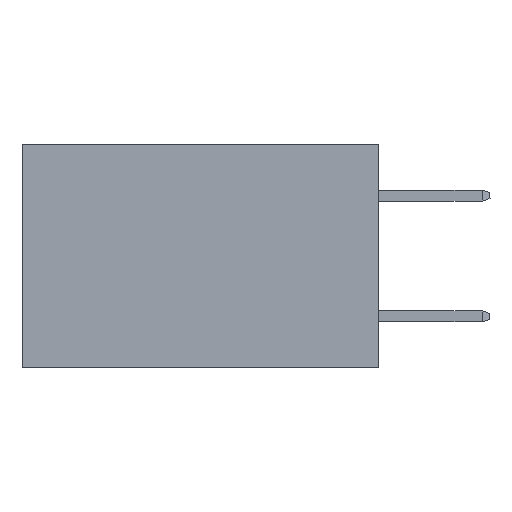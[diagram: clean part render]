
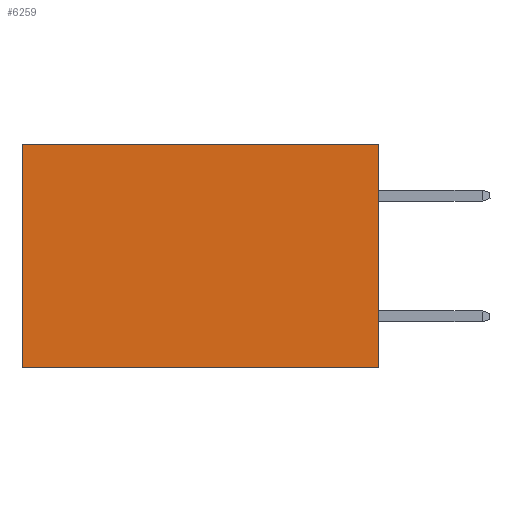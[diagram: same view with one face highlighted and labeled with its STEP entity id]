
A CAD part, left-side view. The second image highlights one B-rep face of the part: STEP entity #6259.
In plain terms, the highlighted planar face has unit normal (-1, 0, 0).
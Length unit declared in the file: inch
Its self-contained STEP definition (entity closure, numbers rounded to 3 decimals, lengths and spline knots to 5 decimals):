
#118 = CARTESIAN_POINT ( 'NONE',  ( 0.277, 0., -0.37 ) ) ;
#153 = EDGE_CURVE ( 'NONE', #3682, #6144, #4287, .T. ) ;
#278 = EDGE_CURVE ( 'NONE', #6315, #3682, #4825, .T. ) ;
#283 = FACE_OUTER_BOUND ( 'NONE', #5601, .T. ) ;
#408 = CARTESIAN_POINT ( 'NONE',  ( 0.277, 0., 0. ) ) ;
#415 = CARTESIAN_POINT ( 'NONE',  ( 0.277, 0., -0.37 ) ) ;
#785 = DIRECTION ( 'NONE',  ( 0., 0., -1. ) ) ;
#802 = VECTOR ( 'NONE', #785, 39.37008 ) ;
#1148 = EDGE_CURVE ( 'NONE', #6315, #6647, #3641, .T. ) ;
#1263 = DIRECTION ( 'NONE',  ( 0., 0., -1. ) ) ;
#1712 = VECTOR ( 'NONE', #2325, 39.37008 ) ;
#1768 = DIRECTION ( 'NONE',  ( 1., 0., 0. ) ) ;
#2311 = CARTESIAN_POINT ( 'NONE',  ( 0.277, 0., 0. ) ) ;
#2325 = DIRECTION ( 'NONE',  ( 0., 1., 0. ) ) ;
#2435 = EDGE_CURVE ( 'NONE', #6647, #6144, #2651, .T. ) ;
#2530 = CARTESIAN_POINT ( 'NONE',  ( 0.277, 0.59, -0.37 ) ) ;
#2597 = AXIS2_PLACEMENT_3D ( 'NONE', #7785, #1768, #6205 ) ;
#2615 = VECTOR ( 'NONE', #3465, 39.37008 ) ;
#2651 = LINE ( 'NONE', #2530, #802 ) ;
#3465 = DIRECTION ( 'NONE',  ( 0., 1., 0. ) ) ;
#3521 = ORIENTED_EDGE ( 'NONE', *, *, #2435, .T. ) ;
#3538 = ORIENTED_EDGE ( 'NONE', *, *, #153, .F. ) ;
#3545 = ORIENTED_EDGE ( 'NONE', *, *, #278, .F. ) ;
#3578 = ORIENTED_EDGE ( 'NONE', *, *, #1148, .T. ) ;
#3641 = LINE ( 'NONE', #2311, #1712 ) ;
#3682 = VERTEX_POINT ( 'NONE', #415 ) ;
#4287 = LINE ( 'NONE', #4395, #2615 ) ;
#4395 = CARTESIAN_POINT ( 'NONE',  ( 0.277, 0., -0.37 ) ) ;
#4825 = LINE ( 'NONE', #118, #7645 ) ;
#4974 = PLANE ( 'NONE',  #2597 ) ;
#5601 = EDGE_LOOP ( 'NONE', ( #3521, #3538, #3545, #3578 ) ) ;
#6144 = VERTEX_POINT ( 'NONE', #7204 ) ;
#6205 = DIRECTION ( 'NONE',  ( 0., 0., -1. ) ) ;
#6259 = ADVANCED_FACE ( 'NONE', ( #283 ), #4974, .F. ) ;
#6315 = VERTEX_POINT ( 'NONE', #408 ) ;
#6647 = VERTEX_POINT ( 'NONE', #6937 ) ;
#6937 = CARTESIAN_POINT ( 'NONE',  ( 0.277, 0.59, 0. ) ) ;
#7204 = CARTESIAN_POINT ( 'NONE',  ( 0.277, 0.59, -0.37 ) ) ;
#7645 = VECTOR ( 'NONE', #1263, 39.37008 ) ;
#7785 = CARTESIAN_POINT ( 'NONE',  ( 0.277, 0., -0.37 ) ) ;
